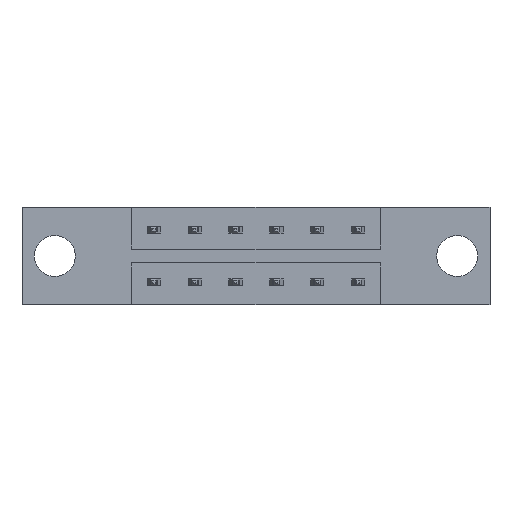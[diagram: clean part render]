
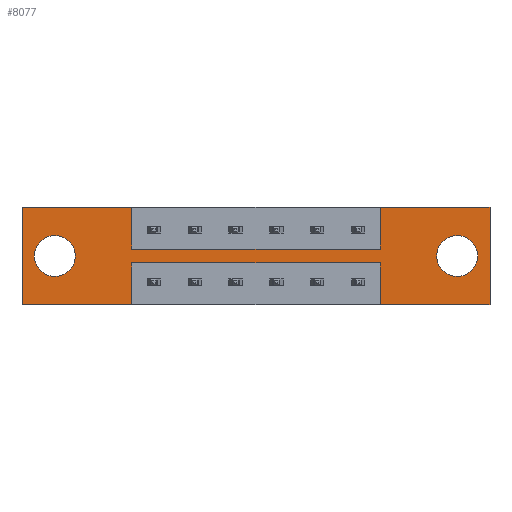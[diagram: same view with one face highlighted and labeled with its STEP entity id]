
A CAD part, front view. The second image highlights one B-rep face of the part: STEP entity #8077.
In plain terms, the highlighted planar face has unit normal (0, -1, 0).
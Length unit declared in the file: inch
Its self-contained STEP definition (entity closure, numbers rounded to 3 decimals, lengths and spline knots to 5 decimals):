
#43 = ORIENTED_EDGE ( 'NONE', *, *, #7920, .F. ) ;
#58 = EDGE_CURVE ( 'NONE', #4217, #4632, #5229, .T. ) ;
#69 = EDGE_LOOP ( 'NONE', ( #1065, #1370 ) ) ;
#79 = VECTOR ( 'NONE', #1520, 39.37008 ) ;
#123 = VERTEX_POINT ( 'NONE', #1503 ) ;
#167 = CARTESIAN_POINT ( 'NONE',  ( 0.4175, 0., -0.1585 ) ) ;
#343 = DIRECTION ( 'NONE',  ( 0., 0., 1. ) ) ;
#346 = CIRCLE ( 'NONE', #1469, 0.078 ) ;
#507 = CARTESIAN_POINT ( 'NONE',  ( 0.4175, 0., -0.1585 ) ) ;
#584 = DIRECTION ( 'NONE',  ( -1., 0., 0. ) ) ;
#595 = DIRECTION ( 'NONE',  ( 1., 0., 0. ) ) ;
#664 = EDGE_CURVE ( 'NONE', #2592, #7519, #5769, .T. ) ;
#668 = EDGE_CURVE ( 'NONE', #3854, #1706, #4577, .T. ) ;
#696 = ORIENTED_EDGE ( 'NONE', *, *, #4981, .F. ) ;
#762 = VECTOR ( 'NONE', #595, 39.37008 ) ;
#773 = CARTESIAN_POINT ( 'NONE',  ( 0.4175, 0., -0.1585 ) ) ;
#787 = AXIS2_PLACEMENT_3D ( 'NONE', #5523, #924, #8155 ) ;
#878 = DIRECTION ( 'NONE',  ( 0., 1., 0. ) ) ;
#904 = EDGE_CURVE ( 'NONE', #8424, #1843, #7931, .T. ) ;
#912 = VERTEX_POINT ( 'NONE', #4826 ) ;
#924 = DIRECTION ( 'NONE',  ( 0., 1., 0. ) ) ;
#958 = ORIENTED_EDGE ( 'NONE', *, *, #6216, .F. ) ;
#1065 = ORIENTED_EDGE ( 'NONE', *, *, #664, .T. ) ;
#1179 = CARTESIAN_POINT ( 'NONE',  ( 0.125, 0., -0.263 ) ) ;
#1240 = EDGE_CURVE ( 'NONE', #2050, #3432, #6075, .T. ) ;
#1341 = DIRECTION ( 'NONE',  ( 0., -1., 0. ) ) ;
#1354 = VECTOR ( 'NONE', #4994, 39.37008 ) ;
#1370 = ORIENTED_EDGE ( 'NONE', *, *, #7836, .T. ) ;
#1424 = FACE_BOUND ( 'NONE', #1934, .T. ) ;
#1469 = AXIS2_PLACEMENT_3D ( 'NONE', #2753, #878, #1506 ) ;
#1503 = CARTESIAN_POINT ( 'NONE',  ( 1.784, 0., 0. ) ) ;
#1506 = DIRECTION ( 'NONE',  ( 0., 0., -1. ) ) ;
#1520 = DIRECTION ( 'NONE',  ( 0., 0., -1. ) ) ;
#1706 = VERTEX_POINT ( 'NONE', #7230 ) ;
#1720 = ORIENTED_EDGE ( 'NONE', *, *, #58, .F. ) ;
#1730 = DIRECTION ( 'NONE',  ( -1., 0., 0. ) ) ;
#1843 = VERTEX_POINT ( 'NONE', #4108 ) ;
#1876 = CARTESIAN_POINT ( 'NONE',  ( 0., 0., -0.37 ) ) ;
#1911 = CARTESIAN_POINT ( 'NONE',  ( 1.784, 0., 0. ) ) ;
#1934 = EDGE_LOOP ( 'NONE', ( #4219, #2812 ) ) ;
#2007 = ORIENTED_EDGE ( 'NONE', *, *, #4374, .F. ) ;
#2050 = VERTEX_POINT ( 'NONE', #5222 ) ;
#2285 = VECTOR ( 'NONE', #1730, 39.37008 ) ;
#2424 = VECTOR ( 'NONE', #2472, 39.37008 ) ;
#2472 = DIRECTION ( 'NONE',  ( 0., 0., -1. ) ) ;
#2592 = VERTEX_POINT ( 'NONE', #8085 ) ;
#2646 = DIRECTION ( 'NONE',  ( 1., 0., 0. ) ) ;
#2726 = CARTESIAN_POINT ( 'NONE',  ( 0.4175, 0., -0.2115 ) ) ;
#2753 = CARTESIAN_POINT ( 'NONE',  ( 1.659, 0., -0.185 ) ) ;
#2766 = FACE_OUTER_BOUND ( 'NONE', #7912, .T. ) ;
#2812 = ORIENTED_EDGE ( 'NONE', *, *, #904, .T. ) ;
#2856 = VECTOR ( 'NONE', #584, 39.37008 ) ;
#2866 = VECTOR ( 'NONE', #3352, 39.37008 ) ;
#3245 = CARTESIAN_POINT ( 'NONE',  ( 1.3665, 0., -0.2115 ) ) ;
#3306 = CARTESIAN_POINT ( 'NONE',  ( 1.3665, 0., -0.1585 ) ) ;
#3318 = VECTOR ( 'NONE', #3385, 39.37008 ) ;
#3352 = DIRECTION ( 'NONE',  ( 1., 0., 0. ) ) ;
#3385 = DIRECTION ( 'NONE',  ( 0., 0., 1. ) ) ;
#3386 = VERTEX_POINT ( 'NONE', #4451 ) ;
#3432 = VERTEX_POINT ( 'NONE', #7002 ) ;
#3471 = LINE ( 'NONE', #773, #4773 ) ;
#3641 = CARTESIAN_POINT ( 'NONE',  ( 0.125, 0., -0.185 ) ) ;
#3825 = CARTESIAN_POINT ( 'NONE',  ( 1.3665, 0., -0.2115 ) ) ;
#3854 = VERTEX_POINT ( 'NONE', #6472 ) ;
#3881 = CARTESIAN_POINT ( 'NONE',  ( 0., 0., -0.37 ) ) ;
#3992 = FACE_BOUND ( 'NONE', #69, .T. ) ;
#4000 = CARTESIAN_POINT ( 'NONE',  ( 0., 0., 0. ) ) ;
#4008 = EDGE_CURVE ( 'NONE', #912, #5707, #4536, .T. ) ;
#4108 = CARTESIAN_POINT ( 'NONE',  ( 1.659, 0., -0.107 ) ) ;
#4217 = VERTEX_POINT ( 'NONE', #3245 ) ;
#4219 = ORIENTED_EDGE ( 'NONE', *, *, #5477, .T. ) ;
#4323 = VERTEX_POINT ( 'NONE', #4723 ) ;
#4374 = EDGE_CURVE ( 'NONE', #4323, #4657, #6021, .T. ) ;
#4386 = CIRCLE ( 'NONE', #5210, 0.078 ) ;
#4451 = CARTESIAN_POINT ( 'NONE',  ( 0., 0., 0. ) ) ;
#4536 = LINE ( 'NONE', #3881, #2856 ) ;
#4550 = CARTESIAN_POINT ( 'NONE',  ( 0., 0., 0. ) ) ;
#4577 = LINE ( 'NONE', #1876, #4935 ) ;
#4632 = VERTEX_POINT ( 'NONE', #5800 ) ;
#4657 = VERTEX_POINT ( 'NONE', #507 ) ;
#4688 = ORIENTED_EDGE ( 'NONE', *, *, #1240, .F. ) ;
#4723 = CARTESIAN_POINT ( 'NONE',  ( 0.4175, 0., 0. ) ) ;
#4737 = ORIENTED_EDGE ( 'NONE', *, *, #4786, .F. ) ;
#4773 = VECTOR ( 'NONE', #2646, 39.37008 ) ;
#4786 = EDGE_CURVE ( 'NONE', #1706, #3386, #6248, .T. ) ;
#4826 = CARTESIAN_POINT ( 'NONE',  ( 1.784, 0., -0.37 ) ) ;
#4873 = ORIENTED_EDGE ( 'NONE', *, *, #668, .F. ) ;
#4935 = VECTOR ( 'NONE', #8369, 39.37008 ) ;
#4981 = EDGE_CURVE ( 'NONE', #3386, #4323, #5994, .T. ) ;
#4994 = DIRECTION ( 'NONE',  ( 0., 0., 1. ) ) ;
#5210 = AXIS2_PLACEMENT_3D ( 'NONE', #3641, #8182, #343 ) ;
#5222 = CARTESIAN_POINT ( 'NONE',  ( 1.3665, 0., -0.1585 ) ) ;
#5229 = LINE ( 'NONE', #6524, #2285 ) ;
#5328 = DIRECTION ( 'NONE',  ( 0., 0., -1. ) ) ;
#5426 = CARTESIAN_POINT ( 'NONE',  ( 1.659, 0., -0.185 ) ) ;
#5449 = PLANE ( 'NONE',  #5598 ) ;
#5465 = DIRECTION ( 'NONE',  ( 0., 0., -1. ) ) ;
#5477 = EDGE_CURVE ( 'NONE', #1843, #8424, #346, .T. ) ;
#5498 = ORIENTED_EDGE ( 'NONE', *, *, #8054, .F. ) ;
#5523 = CARTESIAN_POINT ( 'NONE',  ( 0.125, 0., -0.185 ) ) ;
#5598 = AXIS2_PLACEMENT_3D ( 'NONE', #7997, #1341, #5328 ) ;
#5707 = VERTEX_POINT ( 'NONE', #7044 ) ;
#5769 = CIRCLE ( 'NONE', #787, 0.078 ) ;
#5800 = CARTESIAN_POINT ( 'NONE',  ( 0.4175, 0., -0.2115 ) ) ;
#5882 = AXIS2_PLACEMENT_3D ( 'NONE', #5426, #8050, #5465 ) ;
#5994 = LINE ( 'NONE', #4000, #2866 ) ;
#6021 = LINE ( 'NONE', #167, #6870 ) ;
#6072 = LINE ( 'NONE', #2726, #79 ) ;
#6075 = LINE ( 'NONE', #3306, #3318 ) ;
#6216 = EDGE_CURVE ( 'NONE', #5707, #4217, #6603, .T. ) ;
#6248 = LINE ( 'NONE', #6285, #1354 ) ;
#6285 = CARTESIAN_POINT ( 'NONE',  ( 0., 0., 0. ) ) ;
#6472 = CARTESIAN_POINT ( 'NONE',  ( 0.4175, 0., -0.37 ) ) ;
#6524 = CARTESIAN_POINT ( 'NONE',  ( 0.4175, 0., -0.2115 ) ) ;
#6603 = LINE ( 'NONE', #3825, #6987 ) ;
#6613 = ORIENTED_EDGE ( 'NONE', *, *, #4008, .F. ) ;
#6726 = ORIENTED_EDGE ( 'NONE', *, *, #6948, .F. ) ;
#6870 = VECTOR ( 'NONE', #7388, 39.37008 ) ;
#6939 = ORIENTED_EDGE ( 'NONE', *, *, #8094, .F. ) ;
#6948 = EDGE_CURVE ( 'NONE', #3432, #123, #8259, .T. ) ;
#6987 = VECTOR ( 'NONE', #8502, 39.37008 ) ;
#7002 = CARTESIAN_POINT ( 'NONE',  ( 1.3665, 0., 0. ) ) ;
#7044 = CARTESIAN_POINT ( 'NONE',  ( 1.3665, 0., -0.37 ) ) ;
#7230 = CARTESIAN_POINT ( 'NONE',  ( 0., 0., -0.37 ) ) ;
#7235 = LINE ( 'NONE', #1911, #2424 ) ;
#7388 = DIRECTION ( 'NONE',  ( 0., 0., -1. ) ) ;
#7519 = VERTEX_POINT ( 'NONE', #1179 ) ;
#7772 = CARTESIAN_POINT ( 'NONE',  ( 1.659, 0., -0.263 ) ) ;
#7836 = EDGE_CURVE ( 'NONE', #7519, #2592, #4386, .T. ) ;
#7912 = EDGE_LOOP ( 'NONE', ( #958, #6613, #43, #6726, #4688, #6939, #2007, #696, #4737, #4873, #5498, #1720 ) ) ;
#7920 = EDGE_CURVE ( 'NONE', #123, #912, #7235, .T. ) ;
#7931 = CIRCLE ( 'NONE', #5882, 0.078 ) ;
#7997 = CARTESIAN_POINT ( 'NONE',  ( 0., 0., -0.37 ) ) ;
#8050 = DIRECTION ( 'NONE',  ( 0., 1., 0. ) ) ;
#8054 = EDGE_CURVE ( 'NONE', #4632, #3854, #6072, .T. ) ;
#8077 = ADVANCED_FACE ( 'NONE', ( #1424, #3992, #2766 ), #5449, .T. ) ;
#8085 = CARTESIAN_POINT ( 'NONE',  ( 0.125, 0., -0.107 ) ) ;
#8094 = EDGE_CURVE ( 'NONE', #4657, #2050, #3471, .T. ) ;
#8155 = DIRECTION ( 'NONE',  ( 0., 0., 1. ) ) ;
#8182 = DIRECTION ( 'NONE',  ( 0., 1., 0. ) ) ;
#8259 = LINE ( 'NONE', #4550, #762 ) ;
#8369 = DIRECTION ( 'NONE',  ( -1., 0., 0. ) ) ;
#8424 = VERTEX_POINT ( 'NONE', #7772 ) ;
#8502 = DIRECTION ( 'NONE',  ( 0., 0., 1. ) ) ;
